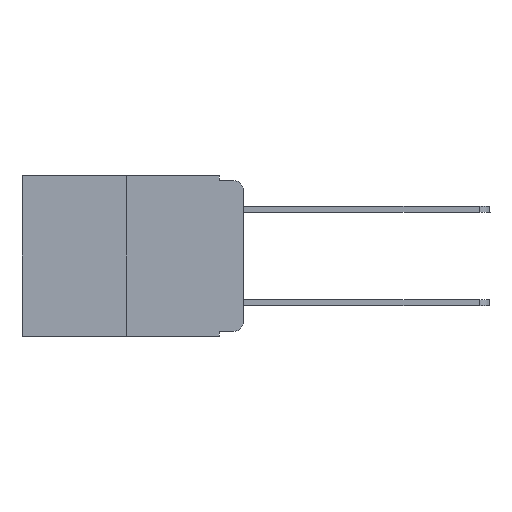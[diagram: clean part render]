
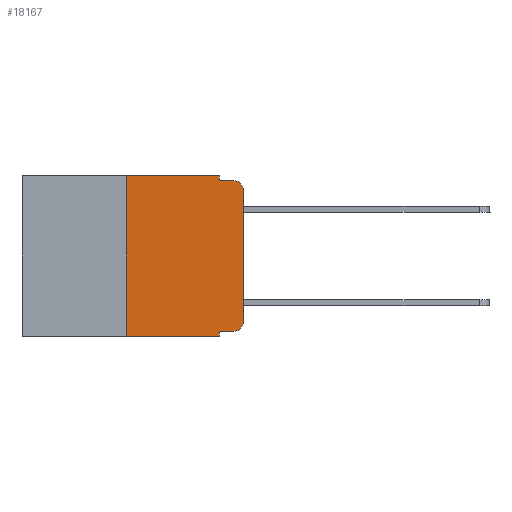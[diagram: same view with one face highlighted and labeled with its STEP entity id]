
A CAD part, left-side view. The second image highlights one B-rep face of the part: STEP entity #18167.
In plain terms, the highlighted planar face has unit normal (-1, 0, 0).
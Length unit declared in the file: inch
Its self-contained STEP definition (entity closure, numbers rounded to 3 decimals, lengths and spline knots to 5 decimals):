
#133 = VERTEX_POINT ( 'NONE', #6235 ) ;
#164 = ORIENTED_EDGE ( 'NONE', *, *, #18489, .T. ) ;
#165 = VERTEX_POINT ( 'NONE', #22491 ) ;
#835 = DIRECTION ( 'NONE',  ( 0., 0., -1. ) ) ;
#916 = ORIENTED_EDGE ( 'NONE', *, *, #5715, .F. ) ;
#1146 = DIRECTION ( 'NONE',  ( 0., -1., 0. ) ) ;
#1256 = ORIENTED_EDGE ( 'NONE', *, *, #20896, .F. ) ;
#1274 = VECTOR ( 'NONE', #13065, 39.37008 ) ;
#1292 = EDGE_CURVE ( 'NONE', #21212, #15838, #1884, .T. ) ;
#1342 = EDGE_LOOP ( 'NONE', ( #15147, #1743, #1603, #21464, #12807, #1256, #13271, #916, #164, #24715 ) ) ;
#1603 = ORIENTED_EDGE ( 'NONE', *, *, #23220, .F. ) ;
#1668 = CARTESIAN_POINT ( 'NONE',  ( 0., 0.051, -0.01 ) ) ;
#1743 = ORIENTED_EDGE ( 'NONE', *, *, #21041, .T. ) ;
#1884 = LINE ( 'NONE', #14934, #16528 ) ;
#2085 = LINE ( 'NONE', #5463, #2345 ) ;
#2184 = CIRCLE ( 'NONE', #14602, 0.02 ) ;
#2345 = VECTOR ( 'NONE', #7717, 39.37008 ) ;
#3139 = DIRECTION ( 'NONE',  ( 1., 0., 0. ) ) ;
#3725 = LINE ( 'NONE', #11355, #21784 ) ;
#5134 = CARTESIAN_POINT ( 'NONE',  ( 0., 0.051, -0.333 ) ) ;
#5463 = CARTESIAN_POINT ( 'NONE',  ( 0., 0., 0. ) ) ;
#5711 = EDGE_CURVE ( 'NONE', #133, #7586, #3725, .T. ) ;
#5715 = EDGE_CURVE ( 'NONE', #11886, #7586, #7612, .T. ) ;
#5763 = EDGE_CURVE ( 'NONE', #165, #9149, #2184, .T. ) ;
#6235 = CARTESIAN_POINT ( 'NONE',  ( 0., 0.25, -0.343 ) ) ;
#6246 = LINE ( 'NONE', #16020, #12818 ) ;
#6348 = DIRECTION ( 'NONE',  ( -1., 0., 0. ) ) ;
#7484 = AXIS2_PLACEMENT_3D ( 'NONE', #9014, #3139, #9268 ) ;
#7586 = VERTEX_POINT ( 'NONE', #13513 ) ;
#7612 = LINE ( 'NONE', #15254, #17773 ) ;
#7717 = DIRECTION ( 'NONE',  ( 0., 0., 1. ) ) ;
#7979 = CARTESIAN_POINT ( 'NONE',  ( 0., 0.02, -0.313 ) ) ;
#8157 = VERTEX_POINT ( 'NONE', #23342 ) ;
#8988 = DIRECTION ( 'NONE',  ( 0., 0., -1. ) ) ;
#9014 = CARTESIAN_POINT ( 'NONE',  ( 0., 0.473, 0. ) ) ;
#9149 = VERTEX_POINT ( 'NONE', #20224 ) ;
#9268 = DIRECTION ( 'NONE',  ( 0., 0., -1. ) ) ;
#9305 = EDGE_CURVE ( 'NONE', #9149, #10299, #2085, .T. ) ;
#10083 = EDGE_CURVE ( 'NONE', #17240, #21212, #12823, .T. ) ;
#10299 = VERTEX_POINT ( 'NONE', #14819 ) ;
#11355 = CARTESIAN_POINT ( 'NONE',  ( 0., 0.473, -0.343 ) ) ;
#11597 = CIRCLE ( 'NONE', #15595, 0.02 ) ;
#11886 = VERTEX_POINT ( 'NONE', #5134 ) ;
#12317 = CARTESIAN_POINT ( 'NONE',  ( 0., 0.473, 0. ) ) ;
#12807 = ORIENTED_EDGE ( 'NONE', *, *, #10083, .F. ) ;
#12818 = VECTOR ( 'NONE', #14402, 39.37008 ) ;
#12823 = LINE ( 'NONE', #12317, #20324 ) ;
#13065 = DIRECTION ( 'NONE',  ( 0., -1., 0. ) ) ;
#13271 = ORIENTED_EDGE ( 'NONE', *, *, #5711, .T. ) ;
#13513 = CARTESIAN_POINT ( 'NONE',  ( 0., 0.051, -0.343 ) ) ;
#14152 = CARTESIAN_POINT ( 'NONE',  ( 0., 0.051, -0.333 ) ) ;
#14396 = CARTESIAN_POINT ( 'NONE',  ( 0., 0.25, 0. ) ) ;
#14402 = DIRECTION ( 'NONE',  ( 0., 0., 1. ) ) ;
#14602 = AXIS2_PLACEMENT_3D ( 'NONE', #7979, #6348, #835 ) ;
#14819 = CARTESIAN_POINT ( 'NONE',  ( 0., 0., -0.03 ) ) ;
#14934 = CARTESIAN_POINT ( 'NONE',  ( 0., 0.051, 0. ) ) ;
#15042 = DIRECTION ( 'NONE',  ( 0., 0., -1. ) ) ;
#15147 = ORIENTED_EDGE ( 'NONE', *, *, #9305, .T. ) ;
#15254 = CARTESIAN_POINT ( 'NONE',  ( 0., 0.051, 0. ) ) ;
#15595 = AXIS2_PLACEMENT_3D ( 'NONE', #22505, #18262, #8988 ) ;
#15838 = VERTEX_POINT ( 'NONE', #1668 ) ;
#16020 = CARTESIAN_POINT ( 'NONE',  ( 0., 0.25, 0. ) ) ;
#16292 = VECTOR ( 'NONE', #23757, 39.37008 ) ;
#16528 = VECTOR ( 'NONE', #15042, 39.37008 ) ;
#17240 = VERTEX_POINT ( 'NONE', #14396 ) ;
#17773 = VECTOR ( 'NONE', #22879, 39.37008 ) ;
#17852 = CARTESIAN_POINT ( 'NONE',  ( 0., 0.051, 0. ) ) ;
#18167 = ADVANCED_FACE ( 'NONE', ( #22528 ), #20262, .F. ) ;
#18262 = DIRECTION ( 'NONE',  ( -1., 0., 0. ) ) ;
#18489 = EDGE_CURVE ( 'NONE', #11886, #165, #19740, .T. ) ;
#18935 = CARTESIAN_POINT ( 'NONE',  ( 0., 0.051, -0.01 ) ) ;
#18989 = DIRECTION ( 'NONE',  ( 0., -1., 0. ) ) ;
#19054 = LINE ( 'NONE', #18935, #1274 ) ;
#19740 = LINE ( 'NONE', #14152, #16292 ) ;
#20224 = CARTESIAN_POINT ( 'NONE',  ( 0., 0., -0.313 ) ) ;
#20262 = PLANE ( 'NONE',  #7484 ) ;
#20324 = VECTOR ( 'NONE', #1146, 39.37008 ) ;
#20896 = EDGE_CURVE ( 'NONE', #133, #17240, #6246, .T. ) ;
#21041 = EDGE_CURVE ( 'NONE', #10299, #8157, #11597, .T. ) ;
#21212 = VERTEX_POINT ( 'NONE', #17852 ) ;
#21464 = ORIENTED_EDGE ( 'NONE', *, *, #1292, .F. ) ;
#21784 = VECTOR ( 'NONE', #18989, 39.37008 ) ;
#22491 = CARTESIAN_POINT ( 'NONE',  ( 0., 0.02, -0.333 ) ) ;
#22505 = CARTESIAN_POINT ( 'NONE',  ( 0., 0.02, -0.03 ) ) ;
#22528 = FACE_OUTER_BOUND ( 'NONE', #1342, .T. ) ;
#22879 = DIRECTION ( 'NONE',  ( 0., 0., -1. ) ) ;
#23220 = EDGE_CURVE ( 'NONE', #15838, #8157, #19054, .T. ) ;
#23342 = CARTESIAN_POINT ( 'NONE',  ( 0., 0.02, -0.01 ) ) ;
#23757 = DIRECTION ( 'NONE',  ( 0., -1., 0. ) ) ;
#24715 = ORIENTED_EDGE ( 'NONE', *, *, #5763, .T. ) ;
